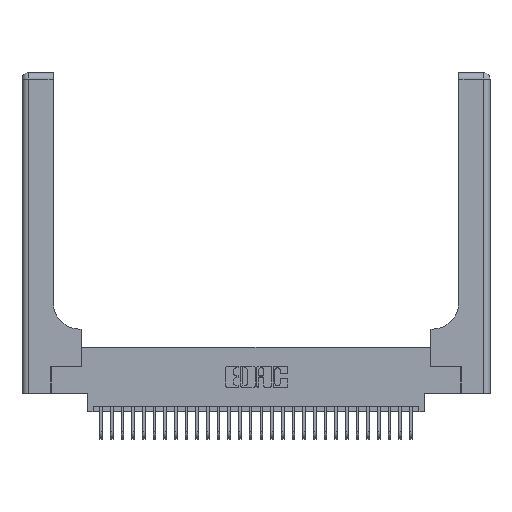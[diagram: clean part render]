
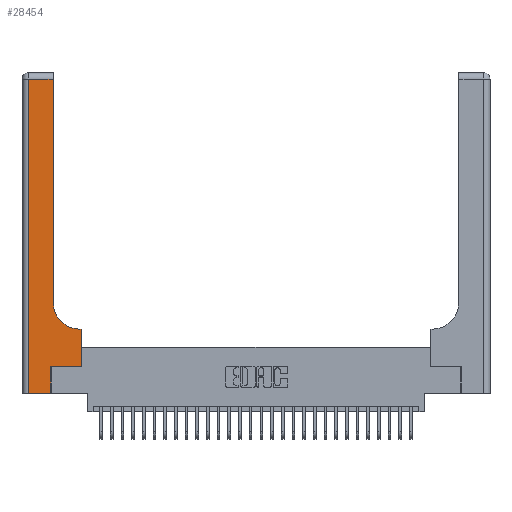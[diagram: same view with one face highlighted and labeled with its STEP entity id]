
A CAD part, top view. The second image highlights one B-rep face of the part: STEP entity #28454.
In plain terms, the highlighted planar face has unit normal (0, 0, 1).
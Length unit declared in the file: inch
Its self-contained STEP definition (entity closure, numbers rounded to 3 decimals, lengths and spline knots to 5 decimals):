
#130 = VERTEX_POINT ( 'NONE', #11959 ) ;
#307 = EDGE_LOOP ( 'NONE', ( #9248, #24859, #30911, #4545, #11554, #5291, #25578, #21455, #17360 ) ) ;
#403 = DIRECTION ( 'NONE',  ( 0., 0., -1. ) ) ;
#1574 = VERTEX_POINT ( 'NONE', #11758 ) ;
#1643 = DIRECTION ( 'NONE',  ( 0., 0., -1. ) ) ;
#1700 = EDGE_CURVE ( 'NONE', #27890, #8197, #28449, .T. ) ;
#2031 = CARTESIAN_POINT ( 'NONE',  ( 0.06, 3., 0.37 ) ) ;
#2436 = EDGE_CURVE ( 'NONE', #15384, #1574, #7276, .T. ) ;
#3328 = CARTESIAN_POINT ( 'NONE',  ( 0.5415, 0.6, 0.37 ) ) ;
#3887 = CARTESIAN_POINT ( 'NONE',  ( 0.2915, 3., 0.37 ) ) ;
#4198 = DIRECTION ( 'NONE',  ( 1., 0., 0. ) ) ;
#4545 = ORIENTED_EDGE ( 'NONE', *, *, #2436, .T. ) ;
#5083 = LINE ( 'NONE', #3887, #26779 ) ;
#5291 = ORIENTED_EDGE ( 'NONE', *, *, #21061, .T. ) ;
#5568 = VERTEX_POINT ( 'NONE', #16985 ) ;
#5984 = CARTESIAN_POINT ( 'NONE',  ( 0.06, 0., 0.37 ) ) ;
#6079 = VECTOR ( 'NONE', #31951, 39.37008 ) ;
#6944 = DIRECTION ( 'NONE',  ( 1., 0., 0. ) ) ;
#7276 = LINE ( 'NONE', #9763, #23904 ) ;
#7551 = DIRECTION ( 'NONE',  ( -1., 0., 0. ) ) ;
#7986 = EDGE_CURVE ( 'NONE', #5568, #21841, #5083, .T. ) ;
#8197 = VERTEX_POINT ( 'NONE', #14387 ) ;
#8984 = VECTOR ( 'NONE', #6944, 39.37008 ) ;
#9248 = ORIENTED_EDGE ( 'NONE', *, *, #7986, .T. ) ;
#9648 = AXIS2_PLACEMENT_3D ( 'NONE', #27681, #403, #7551 ) ;
#9763 = CARTESIAN_POINT ( 'NONE',  ( 0., 0., 0.37 ) ) ;
#10130 = EDGE_CURVE ( 'NONE', #11146, #5568, #25543, .T. ) ;
#10423 = CARTESIAN_POINT ( 'NONE',  ( 0., 2.94, 0.37 ) ) ;
#11146 = VERTEX_POINT ( 'NONE', #3328 ) ;
#11554 = ORIENTED_EDGE ( 'NONE', *, *, #29015, .T. ) ;
#11758 = CARTESIAN_POINT ( 'NONE',  ( 0.269, 0., 0.37 ) ) ;
#11896 = FACE_OUTER_BOUND ( 'NONE', #307, .T. ) ;
#11959 = CARTESIAN_POINT ( 'NONE',  ( 0.06, 2.94, 0.37 ) ) ;
#12086 = DIRECTION ( 'NONE',  ( 0., 1., 0. ) ) ;
#12242 = DIRECTION ( 'NONE',  ( 1., 0., 0. ) ) ;
#13031 = AXIS2_PLACEMENT_3D ( 'NONE', #31358, #1643, #4198 ) ;
#14387 = CARTESIAN_POINT ( 'NONE',  ( 0.5585, 0.6, 0.37 ) ) ;
#14414 = CARTESIAN_POINT ( 'NONE',  ( 0.269, 0.25, 0.37 ) ) ;
#14872 = VECTOR ( 'NONE', #23917, 39.37008 ) ;
#15384 = VERTEX_POINT ( 'NONE', #5984 ) ;
#15598 = VECTOR ( 'NONE', #18199, 39.37008 ) ;
#16411 = VECTOR ( 'NONE', #12086, 39.37008 ) ;
#16985 = CARTESIAN_POINT ( 'NONE',  ( 0.2915, 0.85, 0.37 ) ) ;
#17009 = VECTOR ( 'NONE', #29254, 39.37008 ) ;
#17360 = ORIENTED_EDGE ( 'NONE', *, *, #10130, .T. ) ;
#18199 = DIRECTION ( 'NONE',  ( -1., 0., 0. ) ) ;
#18924 = DIRECTION ( 'NONE',  ( 0., 1., 0. ) ) ;
#19829 = LINE ( 'NONE', #10423, #15598 ) ;
#20037 = EDGE_CURVE ( 'NONE', #8197, #11146, #22620, .T. ) ;
#20713 = EDGE_CURVE ( 'NONE', #21841, #130, #19829, .T. ) ;
#21061 = EDGE_CURVE ( 'NONE', #30098, #27890, #25291, .T. ) ;
#21455 = ORIENTED_EDGE ( 'NONE', *, *, #20037, .T. ) ;
#21841 = VERTEX_POINT ( 'NONE', #31686 ) ;
#22370 = PLANE ( 'NONE',  #9648 ) ;
#22620 = LINE ( 'NONE', #31252, #14872 ) ;
#23049 = CARTESIAN_POINT ( 'NONE',  ( 0.5585, 0.25, 0.37 ) ) ;
#23904 = VECTOR ( 'NONE', #12242, 39.37008 ) ;
#23917 = DIRECTION ( 'NONE',  ( -1., 0., 0. ) ) ;
#23947 = LINE ( 'NONE', #24535, #6079 ) ;
#24535 = CARTESIAN_POINT ( 'NONE',  ( 0.269, 0., 0.37 ) ) ;
#24859 = ORIENTED_EDGE ( 'NONE', *, *, #20713, .T. ) ;
#25291 = LINE ( 'NONE', #14414, #8984 ) ;
#25543 = CIRCLE ( 'NONE', #13031, 0.25 ) ;
#25560 = LINE ( 'NONE', #2031, #17009 ) ;
#25578 = ORIENTED_EDGE ( 'NONE', *, *, #1700, .T. ) ;
#26262 = CARTESIAN_POINT ( 'NONE',  ( 0.269, 0.25, 0.37 ) ) ;
#26779 = VECTOR ( 'NONE', #18924, 39.37008 ) ;
#26934 = CARTESIAN_POINT ( 'NONE',  ( 0.5585, 0.25, 0.37 ) ) ;
#27056 = EDGE_CURVE ( 'NONE', #130, #15384, #25560, .T. ) ;
#27681 = CARTESIAN_POINT ( 'NONE',  ( 0., 3., 0.37 ) ) ;
#27890 = VERTEX_POINT ( 'NONE', #23049 ) ;
#28449 = LINE ( 'NONE', #26934, #16411 ) ;
#28454 = ADVANCED_FACE ( 'NONE', ( #11896 ), #22370, .F. ) ;
#29015 = EDGE_CURVE ( 'NONE', #1574, #30098, #23947, .T. ) ;
#29254 = DIRECTION ( 'NONE',  ( 0., -1., 0. ) ) ;
#30098 = VERTEX_POINT ( 'NONE', #26262 ) ;
#30911 = ORIENTED_EDGE ( 'NONE', *, *, #27056, .T. ) ;
#31252 = CARTESIAN_POINT ( 'NONE',  ( 0.2915, 0.6, 0.37 ) ) ;
#31358 = CARTESIAN_POINT ( 'NONE',  ( 0.5415, 0.85, 0.37 ) ) ;
#31686 = CARTESIAN_POINT ( 'NONE',  ( 0.2915, 2.94, 0.37 ) ) ;
#31951 = DIRECTION ( 'NONE',  ( 0., 1., 0. ) ) ;
